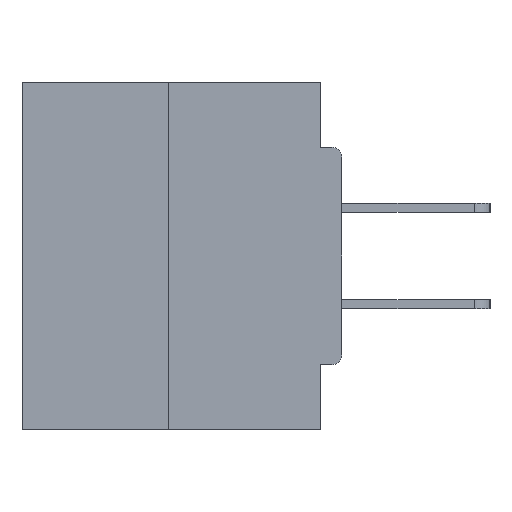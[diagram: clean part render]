
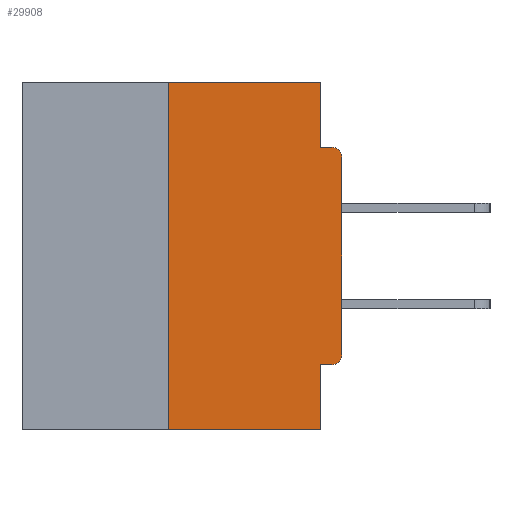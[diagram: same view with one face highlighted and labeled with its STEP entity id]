
A CAD part, left-side view. The second image highlights one B-rep face of the part: STEP entity #29908.
In plain terms, the highlighted planar face has unit normal (-1, 0, 0).
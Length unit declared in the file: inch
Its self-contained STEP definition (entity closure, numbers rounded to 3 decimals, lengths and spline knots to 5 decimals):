
#1738 = VECTOR ( 'NONE', #3461, 39.37008 ) ;
#1840 = VERTEX_POINT ( 'NONE', #26749 ) ;
#2556 = LINE ( 'NONE', #18473, #27614 ) ;
#2802 = VERTEX_POINT ( 'NONE', #14275 ) ;
#2869 = VERTEX_POINT ( 'NONE', #8919 ) ;
#3172 = LINE ( 'NONE', #29299, #5741 ) ;
#3461 = DIRECTION ( 'NONE',  ( 0., 0., 1. ) ) ;
#3874 = AXIS2_PLACEMENT_3D ( 'NONE', #30941, #4782, #33887 ) ;
#4066 = DIRECTION ( 'NONE',  ( 0., 0., -1. ) ) ;
#4151 = CARTESIAN_POINT ( 'NONE',  ( 0., 0.015, -0.0935 ) ) ;
#4579 = DIRECTION ( 'NONE',  ( 0., -1., 0. ) ) ;
#4782 = DIRECTION ( 'NONE',  ( 1., 0., 0. ) ) ;
#5741 = VECTOR ( 'NONE', #11056, 39.37008 ) ;
#6343 = VECTOR ( 'NONE', #28558, 39.37008 ) ;
#6627 = VERTEX_POINT ( 'NONE', #24531 ) ;
#6828 = LINE ( 'NONE', #14423, #20644 ) ;
#8003 = ORIENTED_EDGE ( 'NONE', *, *, #30983, .F. ) ;
#8272 = LINE ( 'NONE', #19222, #1738 ) ;
#8283 = DIRECTION ( 'NONE',  ( 0., 0., -1. ) ) ;
#8798 = DIRECTION ( 'NONE',  ( 0., 0., -1. ) ) ;
#8919 = CARTESIAN_POINT ( 'NONE',  ( 0., 0.031, -0.4065 ) ) ;
#9527 = VERTEX_POINT ( 'NONE', #22525 ) ;
#9894 = CARTESIAN_POINT ( 'NONE',  ( 0., 0.015, -0.3915 ) ) ;
#10028 = EDGE_CURVE ( 'NONE', #10325, #1840, #33734, .T. ) ;
#10302 = FACE_OUTER_BOUND ( 'NONE', #32142, .T. ) ;
#10325 = VERTEX_POINT ( 'NONE', #22468 ) ;
#11000 = EDGE_CURVE ( 'NONE', #31254, #2802, #8272, .T. ) ;
#11056 = DIRECTION ( 'NONE',  ( 0., -1., 0. ) ) ;
#12135 = CARTESIAN_POINT ( 'NONE',  ( 0., 0.031, -0.0935 ) ) ;
#12211 = VECTOR ( 'NONE', #30191, 39.37008 ) ;
#12215 = CARTESIAN_POINT ( 'NONE',  ( 0., 0., 0. ) ) ;
#12602 = CIRCLE ( 'NONE', #17657, 0.015 ) ;
#14275 = CARTESIAN_POINT ( 'NONE',  ( 0., 0.25, 0. ) ) ;
#14334 = LINE ( 'NONE', #27377, #29531 ) ;
#14423 = CARTESIAN_POINT ( 'NONE',  ( 0., 0.46, 0. ) ) ;
#14773 = CARTESIAN_POINT ( 'NONE',  ( 0., 0.015, -0.1085 ) ) ;
#14875 = AXIS2_PLACEMENT_3D ( 'NONE', #14773, #17740, #4066 ) ;
#15222 = ORIENTED_EDGE ( 'NONE', *, *, #33645, .F. ) ;
#15584 = CARTESIAN_POINT ( 'NONE',  ( 0., 0.015, -0.4065 ) ) ;
#16491 = LINE ( 'NONE', #21879, #12211 ) ;
#16584 = ORIENTED_EDGE ( 'NONE', *, *, #29123, .T. ) ;
#17234 = ORIENTED_EDGE ( 'NONE', *, *, #18981, .F. ) ;
#17558 = DIRECTION ( 'NONE',  ( -1., 0., 0. ) ) ;
#17657 = AXIS2_PLACEMENT_3D ( 'NONE', #9894, #17558, #22922 ) ;
#17677 = CIRCLE ( 'NONE', #14875, 0.015 ) ;
#17740 = DIRECTION ( 'NONE',  ( -1., 0., 0. ) ) ;
#17975 = EDGE_CURVE ( 'NONE', #9527, #24515, #14334, .T. ) ;
#18473 = CARTESIAN_POINT ( 'NONE',  ( 0., 0.46, -0.5 ) ) ;
#18981 = EDGE_CURVE ( 'NONE', #2802, #9527, #6828, .T. ) ;
#19222 = CARTESIAN_POINT ( 'NONE',  ( 0., 0.25, 0. ) ) ;
#20247 = ORIENTED_EDGE ( 'NONE', *, *, #20274, .F. ) ;
#20274 = EDGE_CURVE ( 'NONE', #24515, #25067, #3172, .T. ) ;
#20644 = VECTOR ( 'NONE', #4579, 39.37008 ) ;
#21067 = VECTOR ( 'NONE', #8283, 39.37008 ) ;
#21477 = LINE ( 'NONE', #32044, #21067 ) ;
#21879 = CARTESIAN_POINT ( 'NONE',  ( 0., 0., -0.4065 ) ) ;
#22468 = CARTESIAN_POINT ( 'NONE',  ( 0., 0., -0.3915 ) ) ;
#22525 = CARTESIAN_POINT ( 'NONE',  ( 0., 0.031, 0. ) ) ;
#22614 = ORIENTED_EDGE ( 'NONE', *, *, #17975, .F. ) ;
#22922 = DIRECTION ( 'NONE',  ( 0., 0., -1. ) ) ;
#24515 = VERTEX_POINT ( 'NONE', #12135 ) ;
#24531 = CARTESIAN_POINT ( 'NONE',  ( 0., 0.031, -0.5 ) ) ;
#24864 = ORIENTED_EDGE ( 'NONE', *, *, #27122, .T. ) ;
#24977 = ORIENTED_EDGE ( 'NONE', *, *, #10028, .T. ) ;
#25067 = VERTEX_POINT ( 'NONE', #4151 ) ;
#26749 = CARTESIAN_POINT ( 'NONE',  ( 0., 0., -0.1085 ) ) ;
#26892 = EDGE_CURVE ( 'NONE', #31254, #6627, #2556, .T. ) ;
#27122 = EDGE_CURVE ( 'NONE', #1840, #25067, #17677, .T. ) ;
#27377 = CARTESIAN_POINT ( 'NONE',  ( 0., 0.031, 0. ) ) ;
#27614 = VECTOR ( 'NONE', #29053, 39.37008 ) ;
#27679 = VERTEX_POINT ( 'NONE', #15584 ) ;
#28558 = DIRECTION ( 'NONE',  ( 0., 0., 1. ) ) ;
#28689 = PLANE ( 'NONE',  #3874 ) ;
#28860 = CARTESIAN_POINT ( 'NONE',  ( 0., 0.25, -0.5 ) ) ;
#29053 = DIRECTION ( 'NONE',  ( 0., -1., 0. ) ) ;
#29123 = EDGE_CURVE ( 'NONE', #27679, #10325, #12602, .T. ) ;
#29299 = CARTESIAN_POINT ( 'NONE',  ( 0., 0., -0.0935 ) ) ;
#29531 = VECTOR ( 'NONE', #8798, 39.37008 ) ;
#29908 = ADVANCED_FACE ( 'NONE', ( #10302 ), #28689, .F. ) ;
#30191 = DIRECTION ( 'NONE',  ( 0., 1., 0. ) ) ;
#30941 = CARTESIAN_POINT ( 'NONE',  ( 0., 0.46, 0. ) ) ;
#30983 = EDGE_CURVE ( 'NONE', #2869, #6627, #21477, .T. ) ;
#31254 = VERTEX_POINT ( 'NONE', #28860 ) ;
#31635 = ORIENTED_EDGE ( 'NONE', *, *, #11000, .F. ) ;
#32044 = CARTESIAN_POINT ( 'NONE',  ( 0., 0.031, -0.5 ) ) ;
#32082 = ORIENTED_EDGE ( 'NONE', *, *, #26892, .T. ) ;
#32142 = EDGE_LOOP ( 'NONE', ( #17234, #31635, #32082, #8003, #15222, #16584, #24977, #24864, #20247, #22614 ) ) ;
#33645 = EDGE_CURVE ( 'NONE', #27679, #2869, #16491, .T. ) ;
#33734 = LINE ( 'NONE', #12215, #6343 ) ;
#33887 = DIRECTION ( 'NONE',  ( 0., 0., -1. ) ) ;
